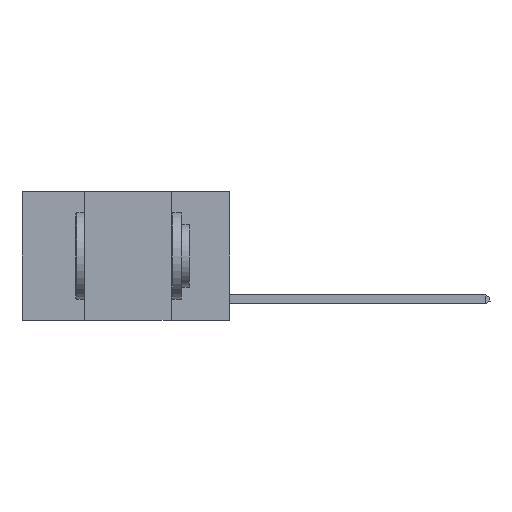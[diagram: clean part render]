
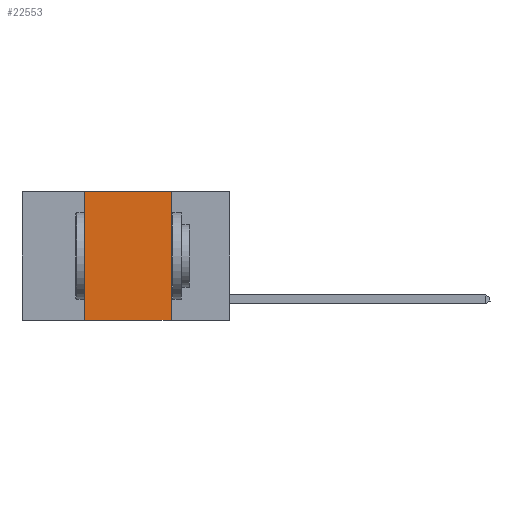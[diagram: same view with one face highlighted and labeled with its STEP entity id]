
A CAD part, left-side view. The second image highlights one B-rep face of the part: STEP entity #22553.
In plain terms, the highlighted planar face has unit normal (-1, 0, 0).
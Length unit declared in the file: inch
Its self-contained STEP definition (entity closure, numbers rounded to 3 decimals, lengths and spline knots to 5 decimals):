
#528 = ORIENTED_EDGE ( 'NONE', *, *, #5017, .F. ) ;
#1048 = VECTOR ( 'NONE', #14058, 39.37008 ) ;
#1586 = ORIENTED_EDGE ( 'NONE', *, *, #10983, .F. ) ;
#2109 = DIRECTION ( 'NONE',  ( 0., 0., 1. ) ) ;
#3021 = CARTESIAN_POINT ( 'NONE',  ( 0., 0.17, -0.37 ) ) ;
#3112 = ORIENTED_EDGE ( 'NONE', *, *, #21039, .T. ) ;
#4068 = ORIENTED_EDGE ( 'NONE', *, *, #7660, .F. ) ;
#4181 = DIRECTION ( 'NONE',  ( 1., 0., 0. ) ) ;
#4185 = LINE ( 'NONE', #22515, #25176 ) ;
#5017 = EDGE_CURVE ( 'NONE', #18240, #16058, #4185, .T. ) ;
#5712 = CARTESIAN_POINT ( 'NONE',  ( 0., 0.6, 0. ) ) ;
#6071 = VECTOR ( 'NONE', #22823, 39.37008 ) ;
#7406 = CARTESIAN_POINT ( 'NONE',  ( 0., 0.42, -0.37 ) ) ;
#7502 = VERTEX_POINT ( 'NONE', #21535 ) ;
#7660 = EDGE_CURVE ( 'NONE', #16058, #7502, #22824, .T. ) ;
#9288 = VECTOR ( 'NONE', #25104, 39.37008 ) ;
#9529 = FACE_OUTER_BOUND ( 'NONE', #22831, .T. ) ;
#10983 = EDGE_CURVE ( 'NONE', #7502, #19403, #22307, .T. ) ;
#14058 = DIRECTION ( 'NONE',  ( 0., -1., 0. ) ) ;
#14490 = CARTESIAN_POINT ( 'NONE',  ( 0., 0.42, 0. ) ) ;
#14509 = CARTESIAN_POINT ( 'NONE',  ( 0., 0.6, 0. ) ) ;
#14772 = LINE ( 'NONE', #17177, #9288 ) ;
#16058 = VERTEX_POINT ( 'NONE', #14490 ) ;
#17177 = CARTESIAN_POINT ( 'NONE',  ( 0., 0.6, -0.37 ) ) ;
#18240 = VERTEX_POINT ( 'NONE', #7406 ) ;
#18550 = DIRECTION ( 'NONE',  ( 0., 0., -1. ) ) ;
#19403 = VERTEX_POINT ( 'NONE', #3021 ) ;
#19612 = AXIS2_PLACEMENT_3D ( 'NONE', #14509, #4181, #18550 ) ;
#20827 = CARTESIAN_POINT ( 'NONE',  ( 0., 0.17, 0. ) ) ;
#21039 = EDGE_CURVE ( 'NONE', #18240, #19403, #14772, .T. ) ;
#21535 = CARTESIAN_POINT ( 'NONE',  ( 0., 0.17, 0. ) ) ;
#22307 = LINE ( 'NONE', #20827, #6071 ) ;
#22515 = CARTESIAN_POINT ( 'NONE',  ( 0., 0.42, 0. ) ) ;
#22553 = ADVANCED_FACE ( 'NONE', ( #9529 ), #24478, .F. ) ;
#22823 = DIRECTION ( 'NONE',  ( 0., 0., -1. ) ) ;
#22824 = LINE ( 'NONE', #5712, #1048 ) ;
#22831 = EDGE_LOOP ( 'NONE', ( #1586, #4068, #528, #3112 ) ) ;
#24478 = PLANE ( 'NONE',  #19612 ) ;
#25104 = DIRECTION ( 'NONE',  ( 0., -1., 0. ) ) ;
#25176 = VECTOR ( 'NONE', #2109, 39.37008 ) ;
